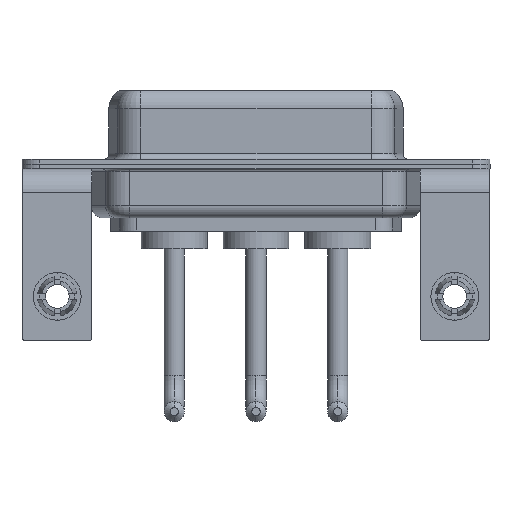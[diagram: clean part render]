
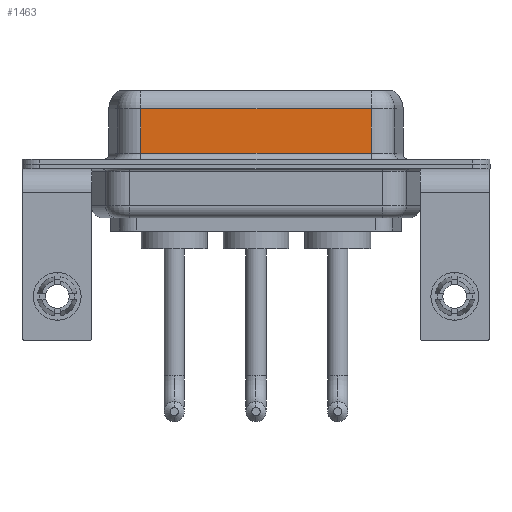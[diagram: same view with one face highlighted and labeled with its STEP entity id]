
A CAD part, front view. The second image highlights one B-rep face of the part: STEP entity #1463.
In plain terms, the highlighted planar face has unit normal (0, -1, 0).
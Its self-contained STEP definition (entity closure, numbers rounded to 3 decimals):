
#33 = DIRECTION ( 'NONE',  ( 0., 0., 1. ) ) ;
#154 = EDGE_CURVE ( 'NONE', #8482, #11285, #1593, .T. ) ;
#1249 = CARTESIAN_POINT ( 'NONE',  ( 26.287, -3.95, 4.65 ) ) ;
#1463 = ADVANCED_FACE ( 'NONE', ( #5551 ), #7988, .F. ) ;
#1593 = LINE ( 'NONE', #7160, #11866 ) ;
#3068 = CARTESIAN_POINT ( 'NONE',  ( 7.013, -3.95, 4.65 ) ) ;
#3295 = ORIENTED_EDGE ( 'NONE', *, *, #9908, .T. ) ;
#3369 = EDGE_CURVE ( 'NONE', #8482, #10227, #11494, .T. ) ;
#3377 = CARTESIAN_POINT ( 'NONE',  ( 26.287, -3.95, 4.65 ) ) ;
#3524 = DIRECTION ( 'NONE',  ( 1., 0., 0. ) ) ;
#4330 = VERTEX_POINT ( 'NONE', #5646 ) ;
#4608 = VECTOR ( 'NONE', #8951, 1000. ) ;
#5425 = ORIENTED_EDGE ( 'NONE', *, *, #154, .F. ) ;
#5551 = FACE_OUTER_BOUND ( 'NONE', #9921, .T. ) ;
#5646 = CARTESIAN_POINT ( 'NONE',  ( 7.013, -3.95, 0.9 ) ) ;
#5703 = EDGE_CURVE ( 'NONE', #10227, #4330, #11363, .T. ) ;
#5801 = CARTESIAN_POINT ( 'NONE',  ( 26.287, -3.95, 0.9 ) ) ;
#6050 = LINE ( 'NONE', #9161, #6446 ) ;
#6446 = VECTOR ( 'NONE', #3524, 1000. ) ;
#7160 = CARTESIAN_POINT ( 'NONE',  ( 26.287, -3.95, 6.4 ) ) ;
#7842 = CARTESIAN_POINT ( 'NONE',  ( 7.013, -3.95, 6.4 ) ) ;
#7988 = PLANE ( 'NONE',  #11680 ) ;
#8482 = VERTEX_POINT ( 'NONE', #1249 ) ;
#8951 = DIRECTION ( 'NONE',  ( 0., 0., -1. ) ) ;
#9097 = DIRECTION ( 'NONE',  ( 0., 1., 0. ) ) ;
#9161 = CARTESIAN_POINT ( 'NONE',  ( 26.287, -3.95, 0.9 ) ) ;
#9243 = CARTESIAN_POINT ( 'NONE',  ( 26.287, -3.95, 6.4 ) ) ;
#9908 = EDGE_CURVE ( 'NONE', #4330, #11285, #6050, .T. ) ;
#9921 = EDGE_LOOP ( 'NONE', ( #5425, #10333, #13537, #3295 ) ) ;
#10227 = VERTEX_POINT ( 'NONE', #3068 ) ;
#10286 = DIRECTION ( 'NONE',  ( -1., 0., 0. ) ) ;
#10333 = ORIENTED_EDGE ( 'NONE', *, *, #3369, .T. ) ;
#10523 = VECTOR ( 'NONE', #10286, 1000. ) ;
#10665 = DIRECTION ( 'NONE',  ( 0., 0., -1. ) ) ;
#11285 = VERTEX_POINT ( 'NONE', #5801 ) ;
#11363 = LINE ( 'NONE', #7842, #4608 ) ;
#11494 = LINE ( 'NONE', #3377, #10523 ) ;
#11680 = AXIS2_PLACEMENT_3D ( 'NONE', #9243, #9097, #33 ) ;
#11866 = VECTOR ( 'NONE', #10665, 1000. ) ;
#13537 = ORIENTED_EDGE ( 'NONE', *, *, #5703, .T. ) ;
